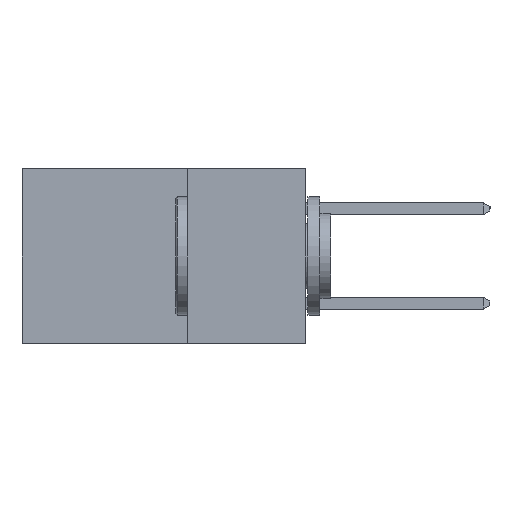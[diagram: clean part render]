
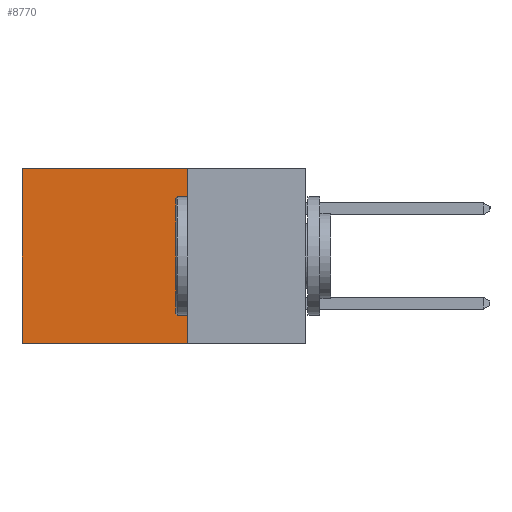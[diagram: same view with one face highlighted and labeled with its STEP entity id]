
A CAD part, left-side view. The second image highlights one B-rep face of the part: STEP entity #8770.
In plain terms, the highlighted planar face has unit normal (-1, 0, 0).
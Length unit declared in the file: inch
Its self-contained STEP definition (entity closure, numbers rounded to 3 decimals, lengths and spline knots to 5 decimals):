
#940 = EDGE_CURVE ( 'NONE', #3855, #3316, #2011, .T. ) ;
#1273 = DIRECTION ( 'NONE',  ( 0., 0., -1. ) ) ;
#1350 = CARTESIAN_POINT ( 'NONE',  ( 0.2615, 0.25, -0.37 ) ) ;
#1501 = EDGE_CURVE ( 'NONE', #11894, #12111, #10331, .T. ) ;
#1877 = VECTOR ( 'NONE', #11232, 39.37008 ) ;
#1916 = ORIENTED_EDGE ( 'NONE', *, *, #2789, .F. ) ;
#2011 = LINE ( 'NONE', #3061, #6132 ) ;
#2066 = CARTESIAN_POINT ( 'NONE',  ( 0.2615, 0.25, -0.37 ) ) ;
#2789 = EDGE_CURVE ( 'NONE', #11894, #3855, #8915, .T. ) ;
#3061 = CARTESIAN_POINT ( 'NONE',  ( 0.2615, 0.25, -0.37 ) ) ;
#3316 = VERTEX_POINT ( 'NONE', #11595 ) ;
#3549 = PLANE ( 'NONE',  #9644 ) ;
#3622 = EDGE_LOOP ( 'NONE', ( #10100, #5673, #1916, #10310 ) ) ;
#3855 = VERTEX_POINT ( 'NONE', #5461 ) ;
#5138 = VECTOR ( 'NONE', #14005, 39.37008 ) ;
#5461 = CARTESIAN_POINT ( 'NONE',  ( 0.2615, 0.25, -0.37 ) ) ;
#5673 = ORIENTED_EDGE ( 'NONE', *, *, #940, .F. ) ;
#5876 = DIRECTION ( 'NONE',  ( 1., 0., 0. ) ) ;
#6132 = VECTOR ( 'NONE', #8929, 39.37008 ) ;
#7029 = CARTESIAN_POINT ( 'NONE',  ( 0.2615, 0.25, 0. ) ) ;
#7172 = CARTESIAN_POINT ( 'NONE',  ( 0.2615, 0.25, 0. ) ) ;
#7735 = DIRECTION ( 'NONE',  ( 0., 0., -1. ) ) ;
#8770 = ADVANCED_FACE ( 'NONE', ( #13590 ), #3549, .F. ) ;
#8915 = LINE ( 'NONE', #2066, #1877 ) ;
#8929 = DIRECTION ( 'NONE',  ( 0., 1., 0. ) ) ;
#8943 = LINE ( 'NONE', #12233, #10192 ) ;
#9644 = AXIS2_PLACEMENT_3D ( 'NONE', #1350, #5876, #1273 ) ;
#10100 = ORIENTED_EDGE ( 'NONE', *, *, #13581, .T. ) ;
#10192 = VECTOR ( 'NONE', #7735, 39.37008 ) ;
#10310 = ORIENTED_EDGE ( 'NONE', *, *, #1501, .T. ) ;
#10331 = LINE ( 'NONE', #7029, #5138 ) ;
#11232 = DIRECTION ( 'NONE',  ( 0., 0., -1. ) ) ;
#11595 = CARTESIAN_POINT ( 'NONE',  ( 0.2615, 0.6, -0.37 ) ) ;
#11894 = VERTEX_POINT ( 'NONE', #7172 ) ;
#12111 = VERTEX_POINT ( 'NONE', #13456 ) ;
#12233 = CARTESIAN_POINT ( 'NONE',  ( 0.2615, 0.6, -0.37 ) ) ;
#13456 = CARTESIAN_POINT ( 'NONE',  ( 0.2615, 0.6, 0. ) ) ;
#13581 = EDGE_CURVE ( 'NONE', #12111, #3316, #8943, .T. ) ;
#13590 = FACE_OUTER_BOUND ( 'NONE', #3622, .T. ) ;
#14005 = DIRECTION ( 'NONE',  ( 0., 1., 0. ) ) ;
